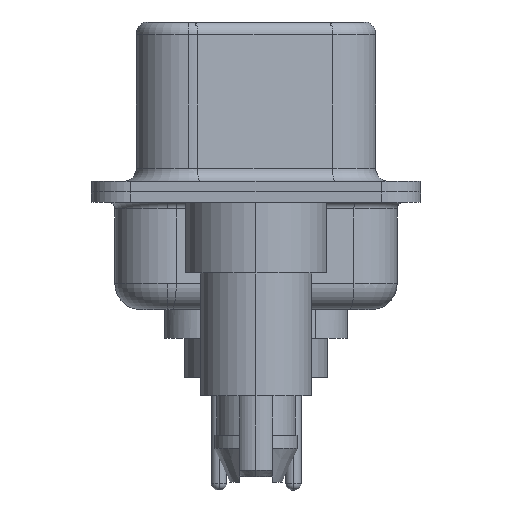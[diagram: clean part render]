
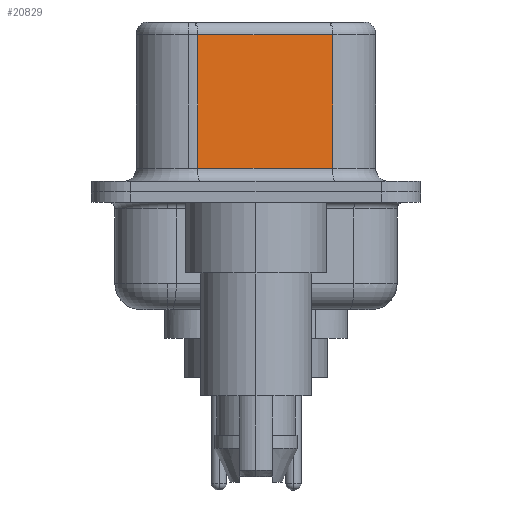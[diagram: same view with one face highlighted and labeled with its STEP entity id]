
A CAD part, left-side view. The second image highlights one B-rep face of the part: STEP entity #20829.
In plain terms, the highlighted planar face has unit normal (-0.985, -0.174, 0).
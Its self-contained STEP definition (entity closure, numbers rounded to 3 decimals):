
#536 = ORIENTED_EDGE ( 'NONE', *, *, #20466, .T. ) ;
#727 = AXIS2_PLACEMENT_3D ( 'NONE', #21989, #3363, #16434 ) ;
#1152 = ORIENTED_EDGE ( 'NONE', *, *, #7699, .T. ) ;
#1546 = CARTESIAN_POINT ( 'NONE',  ( 4.58, -2.927, 6.52 ) ) ;
#1653 = LINE ( 'NONE', #11543, #20939 ) ;
#3002 = LINE ( 'NONE', #1546, #12419 ) ;
#3282 = PLANE ( 'NONE',  #727 ) ;
#3363 = DIRECTION ( 'NONE',  ( 0.985, 0.174, 0. ) ) ;
#5219 = CARTESIAN_POINT ( 'NONE',  ( 3.67, 2.233, 6.02 ) ) ;
#6646 = CARTESIAN_POINT ( 'NONE',  ( 4.58, -2.927, 6.02 ) ) ;
#7699 = EDGE_CURVE ( 'NONE', #14268, #9248, #13273, .T. ) ;
#7785 = DIRECTION ( 'NONE',  ( -0.174, 0.985, 0. ) ) ;
#8355 = VECTOR ( 'NONE', #11477, 1000. ) ;
#9015 = DIRECTION ( 'NONE',  ( 0.174, -0.985, 0. ) ) ;
#9248 = VERTEX_POINT ( 'NONE', #22212 ) ;
#9589 = CARTESIAN_POINT ( 'NONE',  ( 3.67, 2.233, 6.52 ) ) ;
#10756 = VERTEX_POINT ( 'NONE', #18134 ) ;
#11194 = EDGE_LOOP ( 'NONE', ( #14031, #536, #1152, #16359 ) ) ;
#11477 = DIRECTION ( 'NONE',  ( 0., 0., -1. ) ) ;
#11543 = CARTESIAN_POINT ( 'NONE',  ( 4.58, -2.927, 6.02 ) ) ;
#12419 = VECTOR ( 'NONE', #14582, 1000. ) ;
#13273 = LINE ( 'NONE', #9589, #8355 ) ;
#14031 = ORIENTED_EDGE ( 'NONE', *, *, #23987, .F. ) ;
#14268 = VERTEX_POINT ( 'NONE', #5219 ) ;
#14465 = CARTESIAN_POINT ( 'NONE',  ( 4.58, -2.927, 0.9 ) ) ;
#14582 = DIRECTION ( 'NONE',  ( 0., 0., -1. ) ) ;
#16359 = ORIENTED_EDGE ( 'NONE', *, *, #21324, .T. ) ;
#16434 = DIRECTION ( 'NONE',  ( -0.174, 0.985, 0. ) ) ;
#17214 = VERTEX_POINT ( 'NONE', #6646 ) ;
#18134 = CARTESIAN_POINT ( 'NONE',  ( 4.58, -2.927, 0.9 ) ) ;
#18618 = FACE_OUTER_BOUND ( 'NONE', #11194, .T. ) ;
#19188 = VECTOR ( 'NONE', #9015, 1000. ) ;
#20466 = EDGE_CURVE ( 'NONE', #17214, #14268, #1653, .T. ) ;
#20829 = ADVANCED_FACE ( 'NONE', ( #18618 ), #3282, .F. ) ;
#20939 = VECTOR ( 'NONE', #7785, 1000. ) ;
#21324 = EDGE_CURVE ( 'NONE', #9248, #10756, #24123, .T. ) ;
#21989 = CARTESIAN_POINT ( 'NONE',  ( 4.58, -2.927, 6.52 ) ) ;
#22212 = CARTESIAN_POINT ( 'NONE',  ( 3.67, 2.233, 0.9 ) ) ;
#23987 = EDGE_CURVE ( 'NONE', #17214, #10756, #3002, .T. ) ;
#24123 = LINE ( 'NONE', #14465, #19188 ) ;
